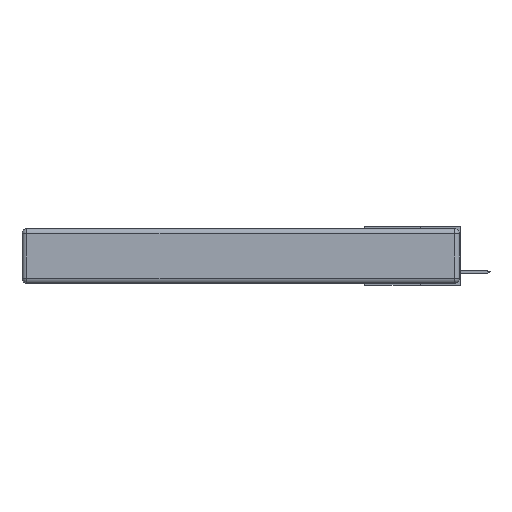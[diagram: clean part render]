
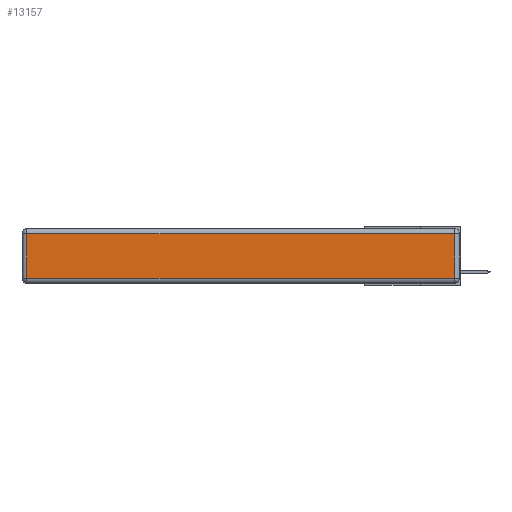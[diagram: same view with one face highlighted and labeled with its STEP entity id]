
A CAD part, left-side view. The second image highlights one B-rep face of the part: STEP entity #13157.
In plain terms, the highlighted planar face has unit normal (-1, 0, 0).
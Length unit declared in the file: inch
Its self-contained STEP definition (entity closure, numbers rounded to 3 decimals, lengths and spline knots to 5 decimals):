
#155 = VECTOR ( 'NONE', #9813, 39.37008 ) ;
#233 = VERTEX_POINT ( 'NONE', #3641 ) ;
#409 = ORIENTED_EDGE ( 'NONE', *, *, #3850, .T. ) ;
#1567 = EDGE_CURVE ( 'NONE', #5160, #233, #12315, .T. ) ;
#2119 = PLANE ( 'NONE',  #3857 ) ;
#3134 = DIRECTION ( 'NONE',  ( -1., 0., 0. ) ) ;
#3641 = CARTESIAN_POINT ( 'NONE',  ( 0., 2.72, -0.313 ) ) ;
#3850 = EDGE_CURVE ( 'NONE', #12801, #5160, #11719, .T. ) ;
#3857 = AXIS2_PLACEMENT_3D ( 'NONE', #13240, #3134, #10291 ) ;
#5160 = VERTEX_POINT ( 'NONE', #6243 ) ;
#5374 = VECTOR ( 'NONE', #13196, 39.37008 ) ;
#5806 = ORIENTED_EDGE ( 'NONE', *, *, #11635, .T. ) ;
#6243 = CARTESIAN_POINT ( 'NONE',  ( 0., 2.72, -0.03 ) ) ;
#6247 = FACE_OUTER_BOUND ( 'NONE', #9978, .T. ) ;
#7255 = VECTOR ( 'NONE', #10056, 39.37008 ) ;
#7628 = CARTESIAN_POINT ( 'NONE',  ( 0., 0.03, -0.343 ) ) ;
#8099 = CARTESIAN_POINT ( 'NONE',  ( 0., 0.03, -0.313 ) ) ;
#8251 = LINE ( 'NONE', #12936, #7255 ) ;
#8715 = EDGE_CURVE ( 'NONE', #13085, #12801, #11995, .T. ) ;
#9196 = CARTESIAN_POINT ( 'NONE',  ( 0., 0.03, -0.03 ) ) ;
#9799 = ORIENTED_EDGE ( 'NONE', *, *, #1567, .T. ) ;
#9813 = DIRECTION ( 'NONE',  ( 0., 0., 1. ) ) ;
#9978 = EDGE_LOOP ( 'NONE', ( #5806, #12041, #409, #9799 ) ) ;
#10003 = CARTESIAN_POINT ( 'NONE',  ( 0., 2.75, -0.03 ) ) ;
#10056 = DIRECTION ( 'NONE',  ( 0., -1., 0. ) ) ;
#10155 = CARTESIAN_POINT ( 'NONE',  ( 0., 2.72, -0.343 ) ) ;
#10188 = DIRECTION ( 'NONE',  ( 0., 1., 0. ) ) ;
#10291 = DIRECTION ( 'NONE',  ( 0., 0., 1. ) ) ;
#11103 = VECTOR ( 'NONE', #10188, 39.37008 ) ;
#11635 = EDGE_CURVE ( 'NONE', #233, #13085, #8251, .T. ) ;
#11719 = LINE ( 'NONE', #10003, #11103 ) ;
#11995 = LINE ( 'NONE', #7628, #155 ) ;
#12041 = ORIENTED_EDGE ( 'NONE', *, *, #8715, .T. ) ;
#12315 = LINE ( 'NONE', #10155, #5374 ) ;
#12801 = VERTEX_POINT ( 'NONE', #9196 ) ;
#12936 = CARTESIAN_POINT ( 'NONE',  ( 0., 0., -0.313 ) ) ;
#13085 = VERTEX_POINT ( 'NONE', #8099 ) ;
#13157 = ADVANCED_FACE ( 'NONE', ( #6247 ), #2119, .T. ) ;
#13196 = DIRECTION ( 'NONE',  ( 0., 0., -1. ) ) ;
#13240 = CARTESIAN_POINT ( 'NONE',  ( 0., 0., -0.343 ) ) ;
